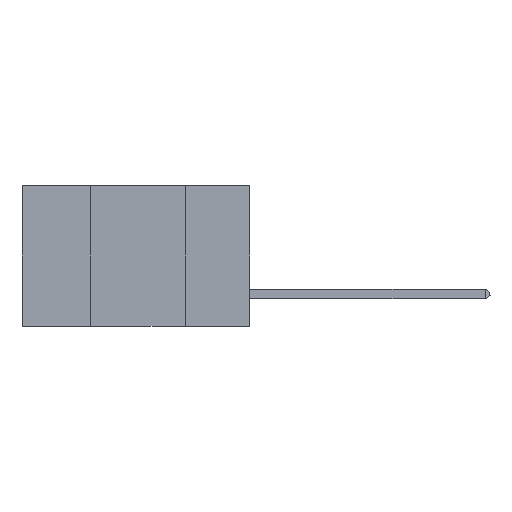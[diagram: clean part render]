
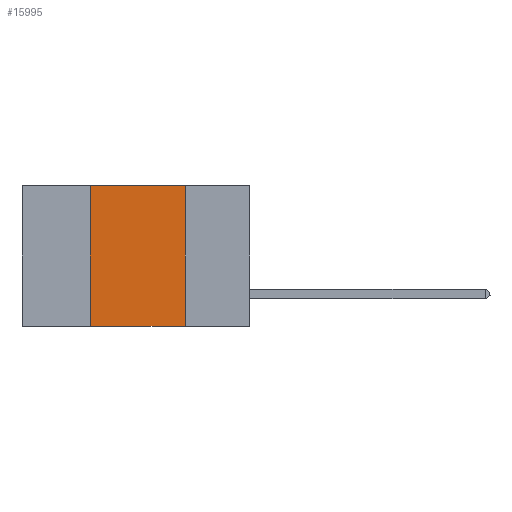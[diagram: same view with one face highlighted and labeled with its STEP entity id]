
A CAD part, left-side view. The second image highlights one B-rep face of the part: STEP entity #15995.
In plain terms, the highlighted planar face has unit normal (-1, 0, 0).
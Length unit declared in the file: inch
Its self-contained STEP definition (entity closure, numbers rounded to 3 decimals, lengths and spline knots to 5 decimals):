
#767 = DIRECTION ( 'NONE',  ( 0., -1., 0. ) ) ;
#810 = VECTOR ( 'NONE', #15939, 39.37008 ) ;
#1216 = EDGE_CURVE ( 'NONE', #4023, #15413, #6496, .T. ) ;
#1265 = LINE ( 'NONE', #7971, #4012 ) ;
#1391 = DIRECTION ( 'NONE',  ( 0., 0., -1. ) ) ;
#2250 = CARTESIAN_POINT ( 'NONE',  ( 0., 0.42, -0.37 ) ) ;
#3001 = AXIS2_PLACEMENT_3D ( 'NONE', #10549, #5383, #1391 ) ;
#3287 = CARTESIAN_POINT ( 'NONE',  ( 0., 0.17, 0. ) ) ;
#4012 = VECTOR ( 'NONE', #4313, 39.37008 ) ;
#4023 = VERTEX_POINT ( 'NONE', #2250 ) ;
#4097 = DIRECTION ( 'NONE',  ( 0., -1., 0. ) ) ;
#4313 = DIRECTION ( 'NONE',  ( 0., 0., -1. ) ) ;
#5383 = DIRECTION ( 'NONE',  ( 1., 0., 0. ) ) ;
#6496 = LINE ( 'NONE', #12011, #810 ) ;
#6652 = EDGE_CURVE ( 'NONE', #9453, #7054, #1265, .T. ) ;
#7054 = VERTEX_POINT ( 'NONE', #10742 ) ;
#7971 = CARTESIAN_POINT ( 'NONE',  ( 0., 0.17, 0. ) ) ;
#9453 = VERTEX_POINT ( 'NONE', #3287 ) ;
#9481 = VECTOR ( 'NONE', #4097, 39.37008 ) ;
#10549 = CARTESIAN_POINT ( 'NONE',  ( 0., 0.6, 0. ) ) ;
#10742 = CARTESIAN_POINT ( 'NONE',  ( 0., 0.17, -0.37 ) ) ;
#11393 = ORIENTED_EDGE ( 'NONE', *, *, #6652, .F. ) ;
#11512 = CARTESIAN_POINT ( 'NONE',  ( 0., 0.42, 0. ) ) ;
#11775 = ORIENTED_EDGE ( 'NONE', *, *, #13507, .F. ) ;
#12011 = CARTESIAN_POINT ( 'NONE',  ( 0., 0.42, 0. ) ) ;
#12165 = CARTESIAN_POINT ( 'NONE',  ( 0., 0.6, 0. ) ) ;
#12239 = EDGE_CURVE ( 'NONE', #4023, #7054, #13037, .T. ) ;
#13037 = LINE ( 'NONE', #14207, #15345 ) ;
#13507 = EDGE_CURVE ( 'NONE', #15413, #9453, #17073, .T. ) ;
#14207 = CARTESIAN_POINT ( 'NONE',  ( 0., 0.6, -0.37 ) ) ;
#14578 = ORIENTED_EDGE ( 'NONE', *, *, #12239, .T. ) ;
#15345 = VECTOR ( 'NONE', #767, 39.37008 ) ;
#15413 = VERTEX_POINT ( 'NONE', #11512 ) ;
#15937 = FACE_OUTER_BOUND ( 'NONE', #17108, .T. ) ;
#15939 = DIRECTION ( 'NONE',  ( 0., 0., 1. ) ) ;
#15995 = ADVANCED_FACE ( 'NONE', ( #15937 ), #17254, .F. ) ;
#16936 = ORIENTED_EDGE ( 'NONE', *, *, #1216, .F. ) ;
#17073 = LINE ( 'NONE', #12165, #9481 ) ;
#17108 = EDGE_LOOP ( 'NONE', ( #11393, #11775, #16936, #14578 ) ) ;
#17254 = PLANE ( 'NONE',  #3001 ) ;
